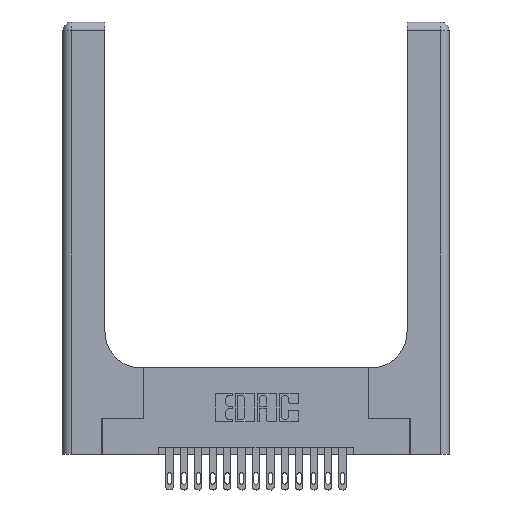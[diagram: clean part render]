
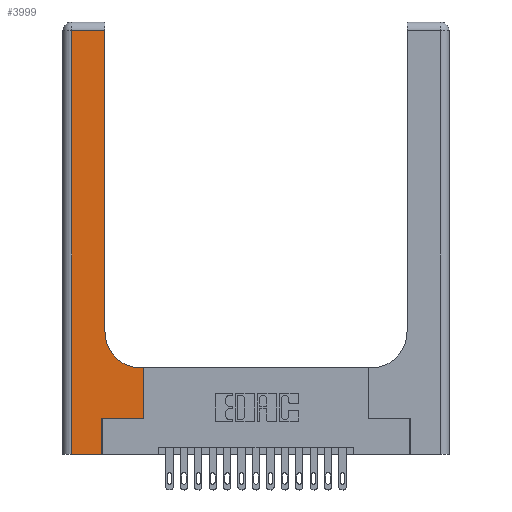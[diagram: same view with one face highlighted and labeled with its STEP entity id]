
A CAD part, top view. The second image highlights one B-rep face of the part: STEP entity #3999.
In plain terms, the highlighted planar face has unit normal (0, 0, 1).
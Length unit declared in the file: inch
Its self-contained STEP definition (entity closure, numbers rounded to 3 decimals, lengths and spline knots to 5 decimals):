
#21 = VERTEX_POINT ( 'NONE', #4324 ) ;
#157 = DIRECTION ( 'NONE',  ( 1., 0., 0. ) ) ;
#510 = ORIENTED_EDGE ( 'NONE', *, *, #16086, .T. ) ;
#629 = CARTESIAN_POINT ( 'NONE',  ( 0.269, 0.25, 0.37 ) ) ;
#764 = DIRECTION ( 'NONE',  ( 0., 1., 0. ) ) ;
#1723 = VERTEX_POINT ( 'NONE', #7751 ) ;
#2021 = DIRECTION ( 'NONE',  ( 0., 1., 0. ) ) ;
#2866 = PLANE ( 'NONE',  #11261 ) ;
#2968 = ORIENTED_EDGE ( 'NONE', *, *, #14087, .T. ) ;
#3250 = EDGE_CURVE ( 'NONE', #1723, #4708, #10756, .T. ) ;
#3468 = VECTOR ( 'NONE', #157, 39.37008 ) ;
#3605 = VECTOR ( 'NONE', #16857, 39.37008 ) ;
#3999 = ADVANCED_FACE ( 'NONE', ( #12125 ), #2866, .F. ) ;
#4033 = CARTESIAN_POINT ( 'NONE',  ( 0.06, 0., 0.37 ) ) ;
#4270 = DIRECTION ( 'NONE',  ( 0., 0., -1. ) ) ;
#4309 = CARTESIAN_POINT ( 'NONE',  ( 0.5585, 0.25, 0.37 ) ) ;
#4324 = CARTESIAN_POINT ( 'NONE',  ( 0.269, 0., 0.37 ) ) ;
#4573 = EDGE_LOOP ( 'NONE', ( #7737, #510, #16074, #19168, #15770, #5121, #6219, #2968, #13551 ) ) ;
#4708 = VERTEX_POINT ( 'NONE', #10631 ) ;
#5016 = CARTESIAN_POINT ( 'NONE',  ( 0.2915, 0.6, 0.37 ) ) ;
#5121 = ORIENTED_EDGE ( 'NONE', *, *, #13783, .T. ) ;
#5147 = CARTESIAN_POINT ( 'NONE',  ( 0.5585, 0.6, 0.37 ) ) ;
#5238 = CARTESIAN_POINT ( 'NONE',  ( 0.06, 2.94, 0.37 ) ) ;
#5382 = EDGE_CURVE ( 'NONE', #8457, #21, #7145, .T. ) ;
#6163 = EDGE_CURVE ( 'NONE', #15904, #7762, #17175, .T. ) ;
#6219 = ORIENTED_EDGE ( 'NONE', *, *, #6163, .T. ) ;
#6364 = CARTESIAN_POINT ( 'NONE',  ( 0.5585, 0.25, 0.37 ) ) ;
#6585 = EDGE_CURVE ( 'NONE', #7625, #8457, #7114, .T. ) ;
#6737 = DIRECTION ( 'NONE',  ( 0., 1., 0. ) ) ;
#6882 = EDGE_CURVE ( 'NONE', #4708, #11795, #18078, .T. ) ;
#7093 = LINE ( 'NONE', #7865, #3605 ) ;
#7114 = LINE ( 'NONE', #14579, #12481 ) ;
#7137 = DIRECTION ( 'NONE',  ( -1., 0., 0. ) ) ;
#7145 = LINE ( 'NONE', #17995, #12058 ) ;
#7228 = EDGE_CURVE ( 'NONE', #21, #13462, #10357, .T. ) ;
#7344 = CARTESIAN_POINT ( 'NONE',  ( 0., 3., 0.37 ) ) ;
#7625 = VERTEX_POINT ( 'NONE', #5238 ) ;
#7737 = ORIENTED_EDGE ( 'NONE', *, *, #6882, .T. ) ;
#7751 = CARTESIAN_POINT ( 'NONE',  ( 0.5415, 0.6, 0.37 ) ) ;
#7762 = VERTEX_POINT ( 'NONE', #5147 ) ;
#7865 = CARTESIAN_POINT ( 'NONE',  ( 0., 2.94, 0.37 ) ) ;
#8175 = DIRECTION ( 'NONE',  ( -1., 0., 0. ) ) ;
#8457 = VERTEX_POINT ( 'NONE', #4033 ) ;
#9049 = DIRECTION ( 'NONE',  ( 1., 0., 0. ) ) ;
#9462 = CARTESIAN_POINT ( 'NONE',  ( 0.2915, 2.94, 0.37 ) ) ;
#9617 = CARTESIAN_POINT ( 'NONE',  ( 0.2915, 3., 0.37 ) ) ;
#9846 = LINE ( 'NONE', #5016, #16609 ) ;
#10227 = CARTESIAN_POINT ( 'NONE',  ( 0.5415, 0.85, 0.37 ) ) ;
#10357 = LINE ( 'NONE', #15462, #16166 ) ;
#10387 = CARTESIAN_POINT ( 'NONE',  ( 0.269, 0.25, 0.37 ) ) ;
#10464 = LINE ( 'NONE', #10387, #3468 ) ;
#10631 = CARTESIAN_POINT ( 'NONE',  ( 0.2915, 0.85, 0.37 ) ) ;
#10756 = CIRCLE ( 'NONE', #16368, 0.25 ) ;
#11261 = AXIS2_PLACEMENT_3D ( 'NONE', #7344, #14831, #7137 ) ;
#11795 = VERTEX_POINT ( 'NONE', #9462 ) ;
#11847 = DIRECTION ( 'NONE',  ( 0., -1., 0. ) ) ;
#11997 = DIRECTION ( 'NONE',  ( 1., 0., 0. ) ) ;
#12058 = VECTOR ( 'NONE', #9049, 39.37008 ) ;
#12125 = FACE_OUTER_BOUND ( 'NONE', #4573, .T. ) ;
#12481 = VECTOR ( 'NONE', #11847, 39.37008 ) ;
#13462 = VERTEX_POINT ( 'NONE', #629 ) ;
#13551 = ORIENTED_EDGE ( 'NONE', *, *, #3250, .T. ) ;
#13783 = EDGE_CURVE ( 'NONE', #13462, #15904, #10464, .T. ) ;
#14087 = EDGE_CURVE ( 'NONE', #7762, #1723, #9846, .T. ) ;
#14579 = CARTESIAN_POINT ( 'NONE',  ( 0.06, 3., 0.37 ) ) ;
#14831 = DIRECTION ( 'NONE',  ( 0., 0., -1. ) ) ;
#15059 = VECTOR ( 'NONE', #2021, 39.37008 ) ;
#15462 = CARTESIAN_POINT ( 'NONE',  ( 0.269, 0., 0.37 ) ) ;
#15731 = VECTOR ( 'NONE', #764, 39.37008 ) ;
#15770 = ORIENTED_EDGE ( 'NONE', *, *, #7228, .T. ) ;
#15904 = VERTEX_POINT ( 'NONE', #4309 ) ;
#16074 = ORIENTED_EDGE ( 'NONE', *, *, #6585, .T. ) ;
#16086 = EDGE_CURVE ( 'NONE', #11795, #7625, #7093, .T. ) ;
#16166 = VECTOR ( 'NONE', #6737, 39.37008 ) ;
#16368 = AXIS2_PLACEMENT_3D ( 'NONE', #10227, #4270, #11997 ) ;
#16609 = VECTOR ( 'NONE', #8175, 39.37008 ) ;
#16857 = DIRECTION ( 'NONE',  ( -1., 0., 0. ) ) ;
#17175 = LINE ( 'NONE', #6364, #15059 ) ;
#17995 = CARTESIAN_POINT ( 'NONE',  ( 0., 0., 0.37 ) ) ;
#18078 = LINE ( 'NONE', #9617, #15731 ) ;
#19168 = ORIENTED_EDGE ( 'NONE', *, *, #5382, .T. ) ;
